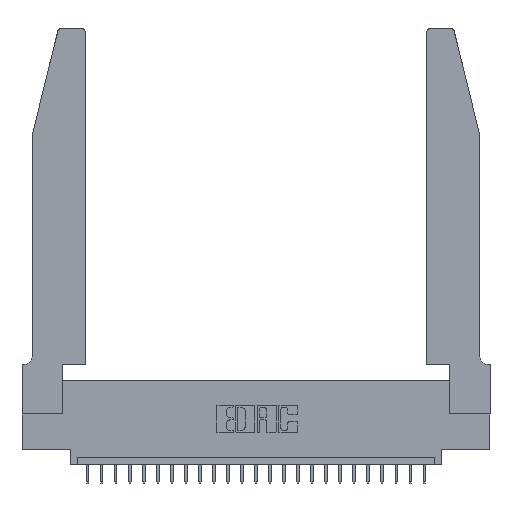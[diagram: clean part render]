
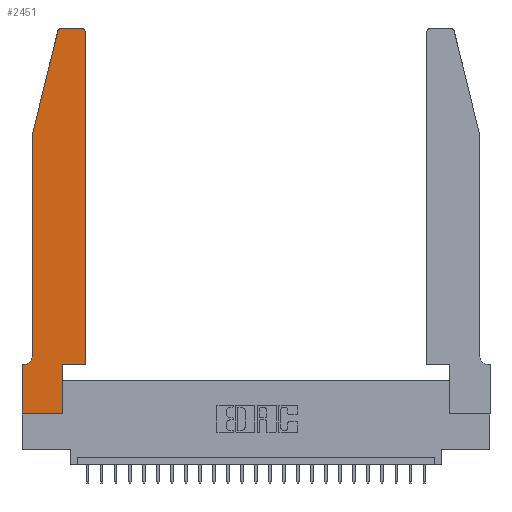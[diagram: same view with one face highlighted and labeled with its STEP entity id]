
A CAD part, top view. The second image highlights one B-rep face of the part: STEP entity #2451.
In plain terms, the highlighted planar face has unit normal (0, 0, 1).
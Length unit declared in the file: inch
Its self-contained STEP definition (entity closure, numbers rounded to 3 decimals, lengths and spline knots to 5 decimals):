
#33 = EDGE_CURVE ( 'NONE', #15192, #12511, #1187, .T. ) ;
#106 = AXIS2_PLACEMENT_3D ( 'NONE', #8570, #20460, #16620 ) ;
#219 = EDGE_CURVE ( 'NONE', #4378, #15192, #7486, .T. ) ;
#742 = LINE ( 'NONE', #24610, #2250 ) ;
#895 = VERTEX_POINT ( 'NONE', #3953 ) ;
#1053 = AXIS2_PLACEMENT_3D ( 'NONE', #21219, #11313, #15643 ) ;
#1187 = LINE ( 'NONE', #9210, #4898 ) ;
#1567 = EDGE_CURVE ( 'NONE', #18354, #8432, #10760, .T. ) ;
#2184 = EDGE_CURVE ( 'NONE', #15626, #21432, #19489, .T. ) ;
#2250 = VECTOR ( 'NONE', #16285, 39.37008 ) ;
#2451 = ADVANCED_FACE ( 'NONE', ( #24554 ), #20988, .T. ) ;
#3161 = LINE ( 'NONE', #15409, #22180 ) ;
#3475 = AXIS2_PLACEMENT_3D ( 'NONE', #15441, #25365, #9639 ) ;
#3708 = CARTESIAN_POINT ( 'NONE',  ( 0.4505, 0.35, 0.37 ) ) ;
#3808 = EDGE_CURVE ( 'NONE', #14568, #23763, #10689, .T. ) ;
#3953 = CARTESIAN_POINT ( 'NONE',  ( 0.284, 2.75, 0.37 ) ) ;
#4378 = VERTEX_POINT ( 'NONE', #24245 ) ;
#4444 = CARTESIAN_POINT ( 'NONE',  ( 0.4205, 2.72, 0.37 ) ) ;
#4873 = DIRECTION ( 'NONE',  ( 1., 0., 0. ) ) ;
#4898 = VECTOR ( 'NONE', #18851, 39.37008 ) ;
#5499 = LINE ( 'NONE', #13149, #16622 ) ;
#6312 = CARTESIAN_POINT ( 'NONE',  ( 0.4505, 0.35, 0.37 ) ) ;
#6332 = ORIENTED_EDGE ( 'NONE', *, *, #2184, .T. ) ;
#7059 = CARTESIAN_POINT ( 'NONE',  ( 0.0055, 0.35, 0.37 ) ) ;
#7464 = CARTESIAN_POINT ( 'NONE',  ( 0.2865, 0., 0.37 ) ) ;
#7486 = LINE ( 'NONE', #15523, #21239 ) ;
#8432 = VERTEX_POINT ( 'NONE', #12403 ) ;
#8503 = EDGE_CURVE ( 'NONE', #23763, #15626, #5499, .T. ) ;
#8504 = EDGE_CURVE ( 'NONE', #895, #14568, #12394, .T. ) ;
#8517 = CARTESIAN_POINT ( 'NONE',  ( 0., 0., 0.37 ) ) ;
#8570 = CARTESIAN_POINT ( 'NONE',  ( 0., 0.35, 0.37 ) ) ;
#8647 = DIRECTION ( 'NONE',  ( 0., -1., 0. ) ) ;
#8924 = EDGE_CURVE ( 'NONE', #16577, #4378, #10505, .T. ) ;
#9210 = CARTESIAN_POINT ( 'NONE',  ( 0.2865, 0.35, 0.37 ) ) ;
#9215 = DIRECTION ( 'NONE',  ( -1., 0., 0. ) ) ;
#9639 = DIRECTION ( 'NONE',  ( -1., 0., 0. ) ) ;
#9898 = AXIS2_PLACEMENT_3D ( 'NONE', #4444, #16049, #24123 ) ;
#9919 = CARTESIAN_POINT ( 'NONE',  ( 0.25487, 2.72718, 0.37 ) ) ;
#10010 = DIRECTION ( 'NONE',  ( 0., 1., 0. ) ) ;
#10166 = ORIENTED_EDGE ( 'NONE', *, *, #10213, .T. ) ;
#10213 = EDGE_CURVE ( 'NONE', #20390, #18354, #20300, .T. ) ;
#10505 = LINE ( 'NONE', #8517, #15783 ) ;
#10689 = LINE ( 'NONE', #10825, #19042 ) ;
#10760 = CIRCLE ( 'NONE', #9898, 0.03 ) ;
#10825 = CARTESIAN_POINT ( 'NONE',  ( 0.0755, 2., 0.37 ) ) ;
#10954 = DIRECTION ( 'NONE',  ( -0.239, -0.971, 0. ) ) ;
#11313 = DIRECTION ( 'NONE',  ( 0., 0., 1. ) ) ;
#12394 = CIRCLE ( 'NONE', #1053, 0.03 ) ;
#12403 = CARTESIAN_POINT ( 'NONE',  ( 0.4205, 2.75, 0.37 ) ) ;
#12477 = ORIENTED_EDGE ( 'NONE', *, *, #33, .T. ) ;
#12511 = VERTEX_POINT ( 'NONE', #13358 ) ;
#12618 = EDGE_LOOP ( 'NONE', ( #22494, #24670, #23347, #19296, #6332, #22633, #16288, #24938, #12477, #12887, #10166, #20590 ) ) ;
#12887 = ORIENTED_EDGE ( 'NONE', *, *, #20650, .T. ) ;
#13142 = EDGE_CURVE ( 'NONE', #8432, #895, #17388, .T. ) ;
#13149 = CARTESIAN_POINT ( 'NONE',  ( 0.0755, 2., 0.37 ) ) ;
#13358 = CARTESIAN_POINT ( 'NONE',  ( 0.2865, 0.35, 0.37 ) ) ;
#14568 = VERTEX_POINT ( 'NONE', #9919 ) ;
#15192 = VERTEX_POINT ( 'NONE', #7464 ) ;
#15409 = CARTESIAN_POINT ( 'NONE',  ( 0.4505, 0.35, 0.37 ) ) ;
#15441 = CARTESIAN_POINT ( 'NONE',  ( 0.0055, 0.42, 0.37 ) ) ;
#15515 = VECTOR ( 'NONE', #9215, 39.37008 ) ;
#15523 = CARTESIAN_POINT ( 'NONE',  ( 0., 0., 0.37 ) ) ;
#15626 = VERTEX_POINT ( 'NONE', #21563 ) ;
#15643 = DIRECTION ( 'NONE',  ( 1., 0., 0. ) ) ;
#15783 = VECTOR ( 'NONE', #8647, 39.37008 ) ;
#15892 = CARTESIAN_POINT ( 'NONE',  ( 0.4505, 2.72, 0.37 ) ) ;
#16049 = DIRECTION ( 'NONE',  ( 0., 0., 1. ) ) ;
#16285 = DIRECTION ( 'NONE',  ( -1., 0., 0. ) ) ;
#16288 = ORIENTED_EDGE ( 'NONE', *, *, #8924, .T. ) ;
#16577 = VERTEX_POINT ( 'NONE', #24008 ) ;
#16620 = DIRECTION ( 'NONE',  ( 1., 0., 0. ) ) ;
#16622 = VECTOR ( 'NONE', #17373, 39.37008 ) ;
#17373 = DIRECTION ( 'NONE',  ( 0., -1., 0. ) ) ;
#17388 = LINE ( 'NONE', #17650, #15515 ) ;
#17650 = CARTESIAN_POINT ( 'NONE',  ( 0.2605, 2.75, 0.37 ) ) ;
#18354 = VERTEX_POINT ( 'NONE', #15892 ) ;
#18522 = DIRECTION ( 'NONE',  ( 1., 0., 0. ) ) ;
#18544 = EDGE_CURVE ( 'NONE', #21432, #16577, #742, .T. ) ;
#18851 = DIRECTION ( 'NONE',  ( 0., 1., 0. ) ) ;
#19042 = VECTOR ( 'NONE', #10954, 39.37008 ) ;
#19296 = ORIENTED_EDGE ( 'NONE', *, *, #8503, .T. ) ;
#19489 = CIRCLE ( 'NONE', #3475, 0.07 ) ;
#20300 = LINE ( 'NONE', #6312, #25139 ) ;
#20390 = VERTEX_POINT ( 'NONE', #3708 ) ;
#20460 = DIRECTION ( 'NONE',  ( 0., 0., 1. ) ) ;
#20590 = ORIENTED_EDGE ( 'NONE', *, *, #1567, .T. ) ;
#20650 = EDGE_CURVE ( 'NONE', #12511, #20390, #3161, .T. ) ;
#20988 = PLANE ( 'NONE',  #106 ) ;
#21219 = CARTESIAN_POINT ( 'NONE',  ( 0.284, 2.72, 0.37 ) ) ;
#21239 = VECTOR ( 'NONE', #18522, 39.37008 ) ;
#21432 = VERTEX_POINT ( 'NONE', #7059 ) ;
#21563 = CARTESIAN_POINT ( 'NONE',  ( 0.0755, 0.42, 0.37 ) ) ;
#22180 = VECTOR ( 'NONE', #4873, 39.37008 ) ;
#22494 = ORIENTED_EDGE ( 'NONE', *, *, #13142, .T. ) ;
#22633 = ORIENTED_EDGE ( 'NONE', *, *, #18544, .T. ) ;
#23347 = ORIENTED_EDGE ( 'NONE', *, *, #3808, .T. ) ;
#23763 = VERTEX_POINT ( 'NONE', #24410 ) ;
#24008 = CARTESIAN_POINT ( 'NONE',  ( 0., 0.35, 0.37 ) ) ;
#24123 = DIRECTION ( 'NONE',  ( 1., 0., 0. ) ) ;
#24245 = CARTESIAN_POINT ( 'NONE',  ( 0., 0., 0.37 ) ) ;
#24410 = CARTESIAN_POINT ( 'NONE',  ( 0.0755, 2., 0.37 ) ) ;
#24554 = FACE_OUTER_BOUND ( 'NONE', #12618, .T. ) ;
#24610 = CARTESIAN_POINT ( 'NONE',  ( 0.0755, 0.35, 0.37 ) ) ;
#24670 = ORIENTED_EDGE ( 'NONE', *, *, #8504, .T. ) ;
#24938 = ORIENTED_EDGE ( 'NONE', *, *, #219, .T. ) ;
#25139 = VECTOR ( 'NONE', #10010, 39.37008 ) ;
#25365 = DIRECTION ( 'NONE',  ( 0., 0., -1. ) ) ;
